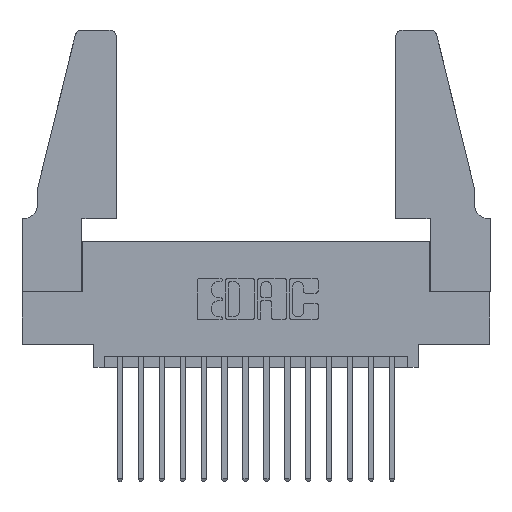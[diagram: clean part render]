
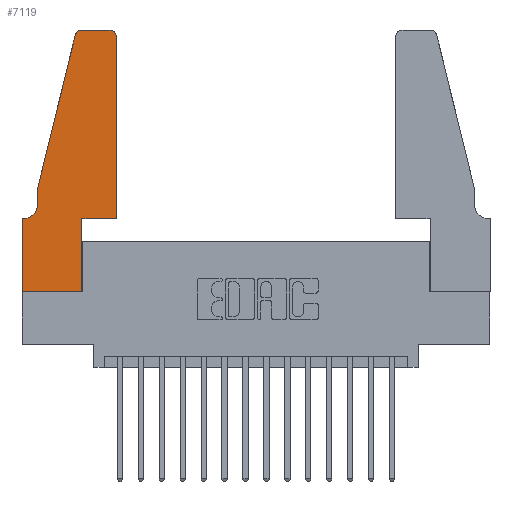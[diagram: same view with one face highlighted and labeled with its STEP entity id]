
A CAD part, top view. The second image highlights one B-rep face of the part: STEP entity #7119.
In plain terms, the highlighted planar face has unit normal (0, 0, 1).
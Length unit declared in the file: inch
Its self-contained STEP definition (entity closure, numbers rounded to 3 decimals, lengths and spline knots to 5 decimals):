
#41 = AXIS2_PLACEMENT_3D ( 'NONE', #367, #1223, #12368 ) ;
#184 = AXIS2_PLACEMENT_3D ( 'NONE', #9227, #1339, #10536 ) ;
#204 = VECTOR ( 'NONE', #14217, 39.37008 ) ;
#206 = VERTEX_POINT ( 'NONE', #8077 ) ;
#253 = DIRECTION ( 'NONE',  ( -0.239, -0.971, 0. ) ) ;
#367 = CARTESIAN_POINT ( 'NONE',  ( 0.0055, 0.42, 0.37 ) ) ;
#432 = CARTESIAN_POINT ( 'NONE',  ( 0.0755, 0.42, 0.37 ) ) ;
#485 = CARTESIAN_POINT ( 'NONE',  ( 0.4505, 0.35, 0.37 ) ) ;
#661 = CARTESIAN_POINT ( 'NONE',  ( 0., 0., 0.37 ) ) ;
#744 = ORIENTED_EDGE ( 'NONE', *, *, #7061, .T. ) ;
#1107 = EDGE_LOOP ( 'NONE', ( #744, #7243, #9858, #6571, #14498, #13177, #5397, #2267, #13928, #2977, #15086, #14406 ) ) ;
#1117 = LINE ( 'NONE', #11177, #4229 ) ;
#1151 = DIRECTION ( 'NONE',  ( 0., 0., 1. ) ) ;
#1223 = DIRECTION ( 'NONE',  ( 0., 0., -1. ) ) ;
#1230 = DIRECTION ( 'NONE',  ( 0., -1., 0. ) ) ;
#1293 = LINE ( 'NONE', #2697, #4357 ) ;
#1339 = DIRECTION ( 'NONE',  ( 0., 0., 1. ) ) ;
#1846 = CIRCLE ( 'NONE', #184, 0.03 ) ;
#2104 = LINE ( 'NONE', #485, #12639 ) ;
#2114 = CARTESIAN_POINT ( 'NONE',  ( 0.4505, 1.22, 0.37 ) ) ;
#2163 = VECTOR ( 'NONE', #9559, 39.37008 ) ;
#2267 = ORIENTED_EDGE ( 'NONE', *, *, #7721, .T. ) ;
#2326 = DIRECTION ( 'NONE',  ( 1., 0., 0. ) ) ;
#2375 = LINE ( 'NONE', #6532, #12509 ) ;
#2446 = CARTESIAN_POINT ( 'NONE',  ( 0.4505, 0.35, 0.37 ) ) ;
#2697 = CARTESIAN_POINT ( 'NONE',  ( 0.0755, 0.5, 0.37 ) ) ;
#2868 = CARTESIAN_POINT ( 'NONE',  ( 0.25487, 1.22718, 0.37 ) ) ;
#2977 = ORIENTED_EDGE ( 'NONE', *, *, #16368, .T. ) ;
#3277 = EDGE_CURVE ( 'NONE', #12129, #16987, #11609, .T. ) ;
#3357 = VERTEX_POINT ( 'NONE', #2868 ) ;
#3637 = CARTESIAN_POINT ( 'NONE',  ( 0.4505, 0.35, 0.37 ) ) ;
#3658 = VERTEX_POINT ( 'NONE', #661 ) ;
#3664 = CARTESIAN_POINT ( 'NONE',  ( 0.4205, 1.22, 0.37 ) ) ;
#4170 = CARTESIAN_POINT ( 'NONE',  ( 0.0755, 0.5, 0.37 ) ) ;
#4229 = VECTOR ( 'NONE', #12517, 39.37008 ) ;
#4357 = VECTOR ( 'NONE', #9265, 39.37008 ) ;
#4529 = VECTOR ( 'NONE', #12913, 39.37008 ) ;
#5006 = DIRECTION ( 'NONE',  ( 1., 0., 0. ) ) ;
#5043 = CARTESIAN_POINT ( 'NONE',  ( 0.2605, 1.25, 0.37 ) ) ;
#5397 = ORIENTED_EDGE ( 'NONE', *, *, #8501, .T. ) ;
#5651 = VERTEX_POINT ( 'NONE', #2114 ) ;
#5680 = LINE ( 'NONE', #12243, #2163 ) ;
#5738 = CARTESIAN_POINT ( 'NONE',  ( 0.4205, 1.25, 0.37 ) ) ;
#6163 = CIRCLE ( 'NONE', #15227, 0.03 ) ;
#6532 = CARTESIAN_POINT ( 'NONE',  ( 0., 0., 0.37 ) ) ;
#6571 = ORIENTED_EDGE ( 'NONE', *, *, #11204, .T. ) ;
#6886 = CARTESIAN_POINT ( 'NONE',  ( 0.0755, 0.5, 0.37 ) ) ;
#7061 = EDGE_CURVE ( 'NONE', #9482, #14757, #16199, .T. ) ;
#7119 = ADVANCED_FACE ( 'NONE', ( #14178 ), #9042, .T. ) ;
#7243 = ORIENTED_EDGE ( 'NONE', *, *, #12532, .T. ) ;
#7721 = EDGE_CURVE ( 'NONE', #3658, #14145, #13953, .T. ) ;
#8077 = CARTESIAN_POINT ( 'NONE',  ( 0.2865, 0.35, 0.37 ) ) ;
#8501 = EDGE_CURVE ( 'NONE', #13861, #3658, #2375, .T. ) ;
#8742 = EDGE_CURVE ( 'NONE', #14145, #206, #5680, .T. ) ;
#9042 = PLANE ( 'NONE',  #13536 ) ;
#9227 = CARTESIAN_POINT ( 'NONE',  ( 0.284, 1.22, 0.37 ) ) ;
#9265 = DIRECTION ( 'NONE',  ( 0., -1., 0. ) ) ;
#9482 = VERTEX_POINT ( 'NONE', #5738 ) ;
#9559 = DIRECTION ( 'NONE',  ( 0., 1., 0. ) ) ;
#9858 = ORIENTED_EDGE ( 'NONE', *, *, #12644, .T. ) ;
#10024 = CARTESIAN_POINT ( 'NONE',  ( 0.284, 1.25, 0.37 ) ) ;
#10216 = CARTESIAN_POINT ( 'NONE',  ( 0., 0., 0.37 ) ) ;
#10356 = DIRECTION ( 'NONE',  ( 1., 0., 0. ) ) ;
#10536 = DIRECTION ( 'NONE',  ( 1., 0., 0. ) ) ;
#10686 = VERTEX_POINT ( 'NONE', #4170 ) ;
#10855 = VECTOR ( 'NONE', #2326, 39.37008 ) ;
#11032 = EDGE_CURVE ( 'NONE', #14268, #5651, #13858, .T. ) ;
#11177 = CARTESIAN_POINT ( 'NONE',  ( 0.0755, 0.35, 0.37 ) ) ;
#11204 = EDGE_CURVE ( 'NONE', #10686, #12129, #1293, .T. ) ;
#11609 = CIRCLE ( 'NONE', #41, 0.07 ) ;
#12129 = VERTEX_POINT ( 'NONE', #432 ) ;
#12243 = CARTESIAN_POINT ( 'NONE',  ( 0.2865, 0.35, 0.37 ) ) ;
#12368 = DIRECTION ( 'NONE',  ( -1., 0., 0. ) ) ;
#12450 = CARTESIAN_POINT ( 'NONE',  ( 0.0055, 0.35, 0.37 ) ) ;
#12509 = VECTOR ( 'NONE', #1230, 39.37008 ) ;
#12517 = DIRECTION ( 'NONE',  ( -1., 0., 0. ) ) ;
#12532 = EDGE_CURVE ( 'NONE', #14757, #3357, #1846, .T. ) ;
#12639 = VECTOR ( 'NONE', #16253, 39.37008 ) ;
#12644 = EDGE_CURVE ( 'NONE', #3357, #10686, #14199, .T. ) ;
#12878 = DIRECTION ( 'NONE',  ( 0., 0., 1. ) ) ;
#12880 = EDGE_CURVE ( 'NONE', #5651, #9482, #6163, .T. ) ;
#12913 = DIRECTION ( 'NONE',  ( -1., 0., 0. ) ) ;
#13177 = ORIENTED_EDGE ( 'NONE', *, *, #15345, .T. ) ;
#13536 = AXIS2_PLACEMENT_3D ( 'NONE', #15569, #1151, #10356 ) ;
#13858 = LINE ( 'NONE', #3637, #204 ) ;
#13861 = VERTEX_POINT ( 'NONE', #16067 ) ;
#13928 = ORIENTED_EDGE ( 'NONE', *, *, #8742, .T. ) ;
#13953 = LINE ( 'NONE', #10216, #10855 ) ;
#14145 = VERTEX_POINT ( 'NONE', #16634 ) ;
#14178 = FACE_OUTER_BOUND ( 'NONE', #1107, .T. ) ;
#14199 = LINE ( 'NONE', #6886, #16840 ) ;
#14217 = DIRECTION ( 'NONE',  ( 0., 1., 0. ) ) ;
#14268 = VERTEX_POINT ( 'NONE', #2446 ) ;
#14406 = ORIENTED_EDGE ( 'NONE', *, *, #12880, .T. ) ;
#14498 = ORIENTED_EDGE ( 'NONE', *, *, #3277, .T. ) ;
#14757 = VERTEX_POINT ( 'NONE', #10024 ) ;
#15086 = ORIENTED_EDGE ( 'NONE', *, *, #11032, .T. ) ;
#15227 = AXIS2_PLACEMENT_3D ( 'NONE', #3664, #12878, #5006 ) ;
#15345 = EDGE_CURVE ( 'NONE', #16987, #13861, #1117, .T. ) ;
#15569 = CARTESIAN_POINT ( 'NONE',  ( 0., 0.35, 0.37 ) ) ;
#16067 = CARTESIAN_POINT ( 'NONE',  ( 0., 0.35, 0.37 ) ) ;
#16199 = LINE ( 'NONE', #5043, #4529 ) ;
#16253 = DIRECTION ( 'NONE',  ( 1., 0., 0. ) ) ;
#16368 = EDGE_CURVE ( 'NONE', #206, #14268, #2104, .T. ) ;
#16634 = CARTESIAN_POINT ( 'NONE',  ( 0.2865, 0., 0.37 ) ) ;
#16840 = VECTOR ( 'NONE', #253, 39.37008 ) ;
#16987 = VERTEX_POINT ( 'NONE', #12450 ) ;
